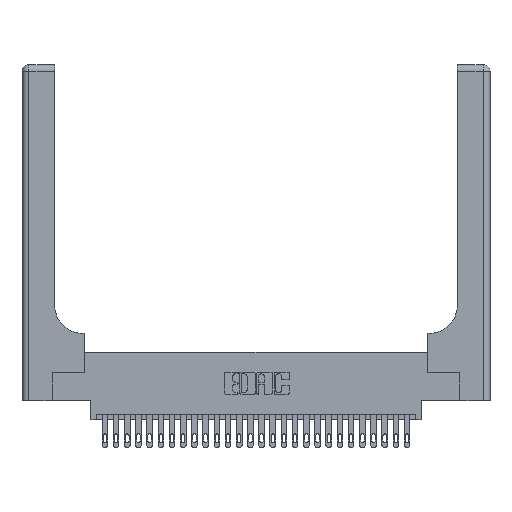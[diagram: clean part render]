
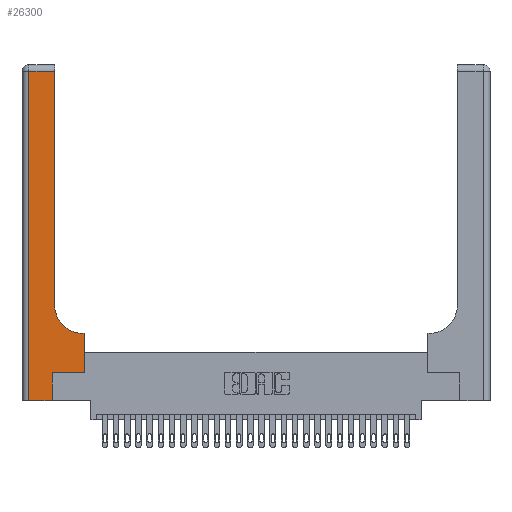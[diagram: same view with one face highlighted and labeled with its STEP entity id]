
A CAD part, top view. The second image highlights one B-rep face of the part: STEP entity #26300.
In plain terms, the highlighted planar face has unit normal (0, 0, 1).
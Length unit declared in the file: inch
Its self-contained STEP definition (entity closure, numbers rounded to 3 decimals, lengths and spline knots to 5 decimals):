
#739 = CARTESIAN_POINT ( 'NONE',  ( 0.2915, 2.94, 0.37 ) ) ;
#1461 = LINE ( 'NONE', #16131, #17952 ) ;
#1636 = LINE ( 'NONE', #4408, #15666 ) ;
#1933 = CARTESIAN_POINT ( 'NONE',  ( 0., 0., 0.37 ) ) ;
#2034 = DIRECTION ( 'NONE',  ( 1., 0., 0. ) ) ;
#2125 = CARTESIAN_POINT ( 'NONE',  ( 0.269, 0.25, 0.37 ) ) ;
#2181 = DIRECTION ( 'NONE',  ( 0., 1., 0. ) ) ;
#2262 = VECTOR ( 'NONE', #15695, 39.37008 ) ;
#2893 = CARTESIAN_POINT ( 'NONE',  ( 0.06, 2.94, 0.37 ) ) ;
#3761 = DIRECTION ( 'NONE',  ( 0., 0., -1. ) ) ;
#4241 = VERTEX_POINT ( 'NONE', #14824 ) ;
#4408 = CARTESIAN_POINT ( 'NONE',  ( 0.06, 3., 0.37 ) ) ;
#5165 = CIRCLE ( 'NONE', #27917, 0.25 ) ;
#5226 = LINE ( 'NONE', #13205, #28817 ) ;
#5874 = PLANE ( 'NONE',  #7100 ) ;
#6356 = VERTEX_POINT ( 'NONE', #2893 ) ;
#6430 = ORIENTED_EDGE ( 'NONE', *, *, #13431, .T. ) ;
#6538 = DIRECTION ( 'NONE',  ( -1., 0., 0. ) ) ;
#6906 = CARTESIAN_POINT ( 'NONE',  ( 0.269, 0., 0.37 ) ) ;
#7100 = AXIS2_PLACEMENT_3D ( 'NONE', #19394, #10421, #19203 ) ;
#7396 = DIRECTION ( 'NONE',  ( 0., 1., 0. ) ) ;
#7619 = CARTESIAN_POINT ( 'NONE',  ( 0.5585, 0.6, 0.37 ) ) ;
#8355 = CARTESIAN_POINT ( 'NONE',  ( 0.269, 0.25, 0.37 ) ) ;
#8789 = DIRECTION ( 'NONE',  ( 1., 0., 0. ) ) ;
#9124 = CARTESIAN_POINT ( 'NONE',  ( 0.269, 0., 0.37 ) ) ;
#9160 = VECTOR ( 'NONE', #8789, 39.37008 ) ;
#9579 = VECTOR ( 'NONE', #7396, 39.37008 ) ;
#9970 = LINE ( 'NONE', #23012, #9579 ) ;
#10421 = DIRECTION ( 'NONE',  ( 0., 0., -1. ) ) ;
#10937 = DIRECTION ( 'NONE',  ( 1., 0., 0. ) ) ;
#11027 = EDGE_LOOP ( 'NONE', ( #27053, #20375, #20225, #28996, #6430, #25651, #24498, #25629, #24579 ) ) ;
#12167 = CARTESIAN_POINT ( 'NONE',  ( 0.5415, 0.6, 0.37 ) ) ;
#12453 = VERTEX_POINT ( 'NONE', #8355 ) ;
#12845 = LINE ( 'NONE', #2125, #16674 ) ;
#13146 = VERTEX_POINT ( 'NONE', #12167 ) ;
#13205 = CARTESIAN_POINT ( 'NONE',  ( 0., 2.94, 0.37 ) ) ;
#13431 = EDGE_CURVE ( 'NONE', #24340, #12453, #22843, .T. ) ;
#14163 = LINE ( 'NONE', #26822, #2262 ) ;
#14824 = CARTESIAN_POINT ( 'NONE',  ( 0.2915, 0.85, 0.37 ) ) ;
#15504 = LINE ( 'NONE', #1933, #9160 ) ;
#15666 = VECTOR ( 'NONE', #20110, 39.37008 ) ;
#15695 = DIRECTION ( 'NONE',  ( -1., 0., 0. ) ) ;
#16131 = CARTESIAN_POINT ( 'NONE',  ( 0.2915, 3., 0.37 ) ) ;
#16346 = EDGE_CURVE ( 'NONE', #6356, #28985, #1636, .T. ) ;
#16591 = VERTEX_POINT ( 'NONE', #739 ) ;
#16638 = CARTESIAN_POINT ( 'NONE',  ( 0.5585, 0.25, 0.37 ) ) ;
#16674 = VECTOR ( 'NONE', #2034, 39.37008 ) ;
#16963 = EDGE_CURVE ( 'NONE', #12453, #23857, #12845, .T. ) ;
#17861 = FACE_OUTER_BOUND ( 'NONE', #11027, .T. ) ;
#17952 = VECTOR ( 'NONE', #23137, 39.37008 ) ;
#18301 = EDGE_CURVE ( 'NONE', #23909, #13146, #14163, .T. ) ;
#19071 = EDGE_CURVE ( 'NONE', #23857, #23909, #9970, .T. ) ;
#19203 = DIRECTION ( 'NONE',  ( -1., 0., 0. ) ) ;
#19394 = CARTESIAN_POINT ( 'NONE',  ( 0., 3., 0.37 ) ) ;
#19535 = EDGE_CURVE ( 'NONE', #4241, #16591, #1461, .T. ) ;
#20002 = EDGE_CURVE ( 'NONE', #28985, #24340, #15504, .T. ) ;
#20110 = DIRECTION ( 'NONE',  ( 0., -1., 0. ) ) ;
#20171 = CARTESIAN_POINT ( 'NONE',  ( 0.06, 0., 0.37 ) ) ;
#20225 = ORIENTED_EDGE ( 'NONE', *, *, #16346, .T. ) ;
#20375 = ORIENTED_EDGE ( 'NONE', *, *, #28782, .T. ) ;
#20423 = EDGE_CURVE ( 'NONE', #13146, #4241, #5165, .T. ) ;
#22843 = LINE ( 'NONE', #9124, #23920 ) ;
#23012 = CARTESIAN_POINT ( 'NONE',  ( 0.5585, 0.25, 0.37 ) ) ;
#23137 = DIRECTION ( 'NONE',  ( 0., 1., 0. ) ) ;
#23857 = VERTEX_POINT ( 'NONE', #16638 ) ;
#23909 = VERTEX_POINT ( 'NONE', #7619 ) ;
#23920 = VECTOR ( 'NONE', #2181, 39.37008 ) ;
#24092 = CARTESIAN_POINT ( 'NONE',  ( 0.5415, 0.85, 0.37 ) ) ;
#24340 = VERTEX_POINT ( 'NONE', #6906 ) ;
#24498 = ORIENTED_EDGE ( 'NONE', *, *, #19071, .T. ) ;
#24579 = ORIENTED_EDGE ( 'NONE', *, *, #20423, .T. ) ;
#25629 = ORIENTED_EDGE ( 'NONE', *, *, #18301, .T. ) ;
#25651 = ORIENTED_EDGE ( 'NONE', *, *, #16963, .T. ) ;
#26300 = ADVANCED_FACE ( 'NONE', ( #17861 ), #5874, .F. ) ;
#26822 = CARTESIAN_POINT ( 'NONE',  ( 0.2915, 0.6, 0.37 ) ) ;
#27053 = ORIENTED_EDGE ( 'NONE', *, *, #19535, .T. ) ;
#27917 = AXIS2_PLACEMENT_3D ( 'NONE', #24092, #3761, #10937 ) ;
#28782 = EDGE_CURVE ( 'NONE', #16591, #6356, #5226, .T. ) ;
#28817 = VECTOR ( 'NONE', #6538, 39.37008 ) ;
#28985 = VERTEX_POINT ( 'NONE', #20171 ) ;
#28996 = ORIENTED_EDGE ( 'NONE', *, *, #20002, .T. ) ;
